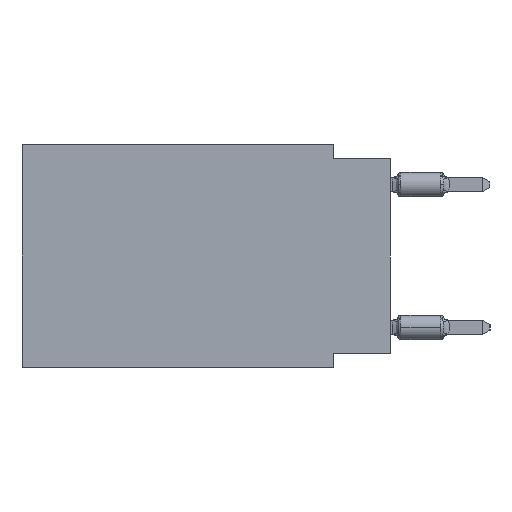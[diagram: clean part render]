
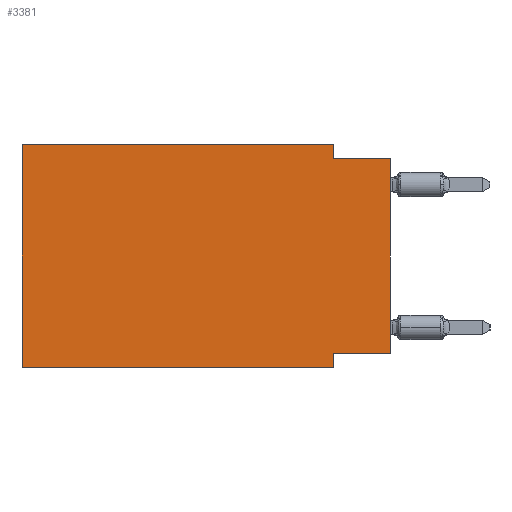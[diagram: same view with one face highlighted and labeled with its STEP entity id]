
A CAD part, left-side view. The second image highlights one B-rep face of the part: STEP entity #3381.
In plain terms, the highlighted planar face has unit normal (-1, 0, 0).
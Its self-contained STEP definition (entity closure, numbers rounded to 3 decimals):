
#170 = CARTESIAN_POINT ( 'NONE',  ( 0., 2.54, -9.906 ) ) ;
#388 = CARTESIAN_POINT ( 'NONE',  ( 0., 16.383, 0. ) ) ;
#711 = VERTEX_POINT ( 'NONE', #28777 ) ;
#888 = LINE ( 'NONE', #17311, #3138 ) ;
#1368 = DIRECTION ( 'NONE',  ( 0., -1., 0. ) ) ;
#1557 = CARTESIAN_POINT ( 'NONE',  ( 0., 16.383, 0. ) ) ;
#1678 = LINE ( 'NONE', #19464, #11044 ) ;
#1712 = ORIENTED_EDGE ( 'NONE', *, *, #9049, .F. ) ;
#3138 = VECTOR ( 'NONE', #28746, 1000. ) ;
#3381 = ADVANCED_FACE ( 'NONE', ( #20523 ), #9217, .F. ) ;
#3419 = DIRECTION ( 'NONE',  ( 0., 1., 0. ) ) ;
#3563 = VECTOR ( 'NONE', #22203, 1000. ) ;
#4306 = VERTEX_POINT ( 'NONE', #26701 ) ;
#4802 = ORIENTED_EDGE ( 'NONE', *, *, #15129, .F. ) ;
#5041 = VERTEX_POINT ( 'NONE', #10203 ) ;
#5216 = VERTEX_POINT ( 'NONE', #388 ) ;
#6296 = VERTEX_POINT ( 'NONE', #25419 ) ;
#6429 = DIRECTION ( 'NONE',  ( 0., 0., -1. ) ) ;
#7135 = CARTESIAN_POINT ( 'NONE',  ( 0., 16.383, 0. ) ) ;
#9049 = EDGE_CURVE ( 'NONE', #4306, #9832, #10786, .T. ) ;
#9217 = PLANE ( 'NONE',  #28854 ) ;
#9465 = DIRECTION ( 'NONE',  ( 0., -1., 0. ) ) ;
#9792 = VECTOR ( 'NONE', #22172, 1000. ) ;
#9832 = VERTEX_POINT ( 'NONE', #170 ) ;
#10102 = ORIENTED_EDGE ( 'NONE', *, *, #27021, .T. ) ;
#10203 = CARTESIAN_POINT ( 'NONE',  ( 0., 0., -0.635 ) ) ;
#10463 = LINE ( 'NONE', #1557, #3563 ) ;
#10469 = EDGE_CURVE ( 'NONE', #12317, #5041, #888, .T. ) ;
#10786 = LINE ( 'NONE', #19984, #24737 ) ;
#11044 = VECTOR ( 'NONE', #12998, 1000. ) ;
#11834 = CARTESIAN_POINT ( 'NONE',  ( 0., 0., -9.271 ) ) ;
#12317 = VERTEX_POINT ( 'NONE', #11834 ) ;
#12998 = DIRECTION ( 'NONE',  ( 0., 0., -1. ) ) ;
#13256 = LINE ( 'NONE', #25440, #21107 ) ;
#13756 = DIRECTION ( 'NONE',  ( 1., 0., 0. ) ) ;
#14019 = EDGE_CURVE ( 'NONE', #5216, #711, #13256, .T. ) ;
#15129 = EDGE_CURVE ( 'NONE', #711, #6296, #1678, .T. ) ;
#15701 = ORIENTED_EDGE ( 'NONE', *, *, #10469, .T. ) ;
#15907 = EDGE_CURVE ( 'NONE', #16140, #5216, #10463, .T. ) ;
#16140 = VERTEX_POINT ( 'NONE', #27770 ) ;
#17244 = ORIENTED_EDGE ( 'NONE', *, *, #26616, .F. ) ;
#17311 = CARTESIAN_POINT ( 'NONE',  ( 0., 0., 0. ) ) ;
#17972 = ORIENTED_EDGE ( 'NONE', *, *, #14019, .F. ) ;
#19464 = CARTESIAN_POINT ( 'NONE',  ( 0., 2.54, 0. ) ) ;
#19608 = CARTESIAN_POINT ( 'NONE',  ( 0., 0., -0.635 ) ) ;
#19984 = CARTESIAN_POINT ( 'NONE',  ( 0., 2.54, -9.906 ) ) ;
#20063 = CARTESIAN_POINT ( 'NONE',  ( 0., 16.383, -9.906 ) ) ;
#20212 = LINE ( 'NONE', #20063, #9792 ) ;
#20278 = ORIENTED_EDGE ( 'NONE', *, *, #15907, .F. ) ;
#20523 = FACE_OUTER_BOUND ( 'NONE', #25777, .T. ) ;
#20956 = EDGE_CURVE ( 'NONE', #6296, #5041, #21425, .T. ) ;
#20973 = DIRECTION ( 'NONE',  ( 0., 0., -1. ) ) ;
#21107 = VECTOR ( 'NONE', #9465, 1000. ) ;
#21425 = LINE ( 'NONE', #19608, #26657 ) ;
#22172 = DIRECTION ( 'NONE',  ( 0., -1., 0. ) ) ;
#22203 = DIRECTION ( 'NONE',  ( 0., 0., 1. ) ) ;
#23140 = ORIENTED_EDGE ( 'NONE', *, *, #20956, .F. ) ;
#24373 = LINE ( 'NONE', #26317, #27050 ) ;
#24737 = VECTOR ( 'NONE', #6429, 1000. ) ;
#25419 = CARTESIAN_POINT ( 'NONE',  ( 0., 2.54, -0.635 ) ) ;
#25440 = CARTESIAN_POINT ( 'NONE',  ( 0., 16.383, 0. ) ) ;
#25777 = EDGE_LOOP ( 'NONE', ( #15701, #23140, #4802, #17972, #20278, #10102, #1712, #17244 ) ) ;
#26317 = CARTESIAN_POINT ( 'NONE',  ( 0., 0., -9.271 ) ) ;
#26616 = EDGE_CURVE ( 'NONE', #12317, #4306, #24373, .T. ) ;
#26657 = VECTOR ( 'NONE', #1368, 1000. ) ;
#26701 = CARTESIAN_POINT ( 'NONE',  ( 0., 2.54, -9.271 ) ) ;
#27021 = EDGE_CURVE ( 'NONE', #16140, #9832, #20212, .T. ) ;
#27050 = VECTOR ( 'NONE', #3419, 1000. ) ;
#27770 = CARTESIAN_POINT ( 'NONE',  ( 0., 16.383, -9.906 ) ) ;
#28746 = DIRECTION ( 'NONE',  ( 0., 0., 1. ) ) ;
#28777 = CARTESIAN_POINT ( 'NONE',  ( 0., 2.54, 0. ) ) ;
#28854 = AXIS2_PLACEMENT_3D ( 'NONE', #7135, #13756, #20973 ) ;
